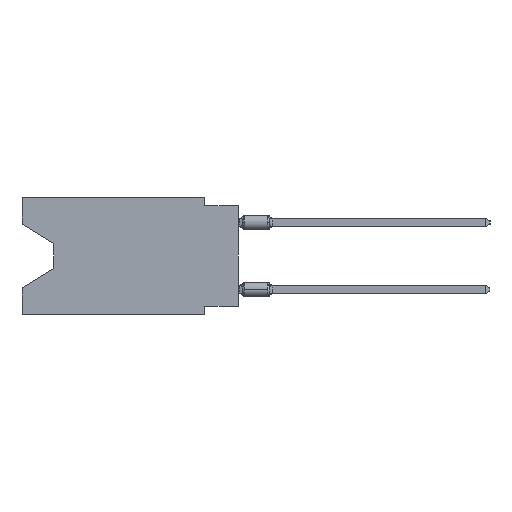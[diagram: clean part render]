
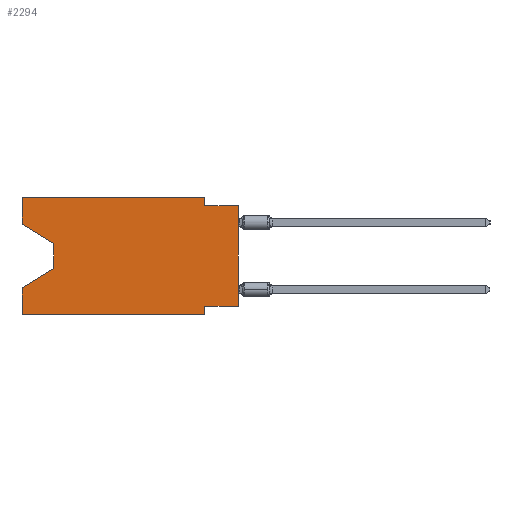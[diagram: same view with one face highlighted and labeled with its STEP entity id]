
A CAD part, left-side view. The second image highlights one B-rep face of the part: STEP entity #2294.
In plain terms, the highlighted planar face has unit normal (-1, 0, 0).
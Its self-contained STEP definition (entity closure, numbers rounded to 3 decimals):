
#181 = ORIENTED_EDGE ( 'NONE', *, *, #17903, .F. ) ;
#265 = LINE ( 'NONE', #28684, #13404 ) ;
#426 = VERTEX_POINT ( 'NONE', #13703 ) ;
#1508 = EDGE_CURVE ( 'NONE', #11609, #426, #4646, .T. ) ;
#1992 = ORIENTED_EDGE ( 'NONE', *, *, #17382, .T. ) ;
#2086 = ORIENTED_EDGE ( 'NONE', *, *, #25789, .F. ) ;
#2294 = ADVANCED_FACE ( 'NONE', ( #4104 ), #13522, .F. ) ;
#2519 = CARTESIAN_POINT ( 'NONE',  ( 0., 16.383, -8.89 ) ) ;
#3212 = VERTEX_POINT ( 'NONE', #23504 ) ;
#3384 = EDGE_CURVE ( 'NONE', #19287, #3212, #8581, .T. ) ;
#4104 = FACE_OUTER_BOUND ( 'NONE', #4365, .T. ) ;
#4188 = EDGE_CURVE ( 'NONE', #10632, #11609, #29544, .T. ) ;
#4365 = EDGE_LOOP ( 'NONE', ( #20825, #10486, #22707, #2086, #10446, #16265, #16958, #1992, #13049, #181, #12769, #13996 ) ) ;
#4429 = CARTESIAN_POINT ( 'NONE',  ( 0., 0., -8.255 ) ) ;
#4646 = LINE ( 'NONE', #26424, #22206 ) ;
#5710 = VERTEX_POINT ( 'NONE', #7734 ) ;
#6050 = CARTESIAN_POINT ( 'NONE',  ( 0., 13.97, -3.505 ) ) ;
#6409 = CARTESIAN_POINT ( 'NONE',  ( 0., 16.383, 0. ) ) ;
#6867 = VERTEX_POINT ( 'NONE', #6409 ) ;
#7337 = DIRECTION ( 'NONE',  ( 0., 0., -1. ) ) ;
#7412 = DIRECTION ( 'NONE',  ( 0., 0.855, -0.519 ) ) ;
#7734 = CARTESIAN_POINT ( 'NONE',  ( 0., 2.54, -0.635 ) ) ;
#8309 = VECTOR ( 'NONE', #18363, 1000. ) ;
#8549 = LINE ( 'NONE', #27427, #27385 ) ;
#8566 = EDGE_CURVE ( 'NONE', #23685, #6867, #21553, .T. ) ;
#8581 = LINE ( 'NONE', #22816, #19250 ) ;
#10019 = CARTESIAN_POINT ( 'NONE',  ( 0., 0., -0.635 ) ) ;
#10324 = LINE ( 'NONE', #10019, #10648 ) ;
#10446 = ORIENTED_EDGE ( 'NONE', *, *, #27778, .T. ) ;
#10486 = ORIENTED_EDGE ( 'NONE', *, *, #4188, .T. ) ;
#10632 = VERTEX_POINT ( 'NONE', #27458 ) ;
#10648 = VECTOR ( 'NONE', #22377, 1000. ) ;
#10943 = LINE ( 'NONE', #29951, #8309 ) ;
#11191 = CARTESIAN_POINT ( 'NONE',  ( 0., 2.54, 0. ) ) ;
#11609 = VERTEX_POINT ( 'NONE', #29880 ) ;
#11934 = DIRECTION ( 'NONE',  ( 0., -1., 0. ) ) ;
#12244 = LINE ( 'NONE', #22530, #25513 ) ;
#12429 = CARTESIAN_POINT ( 'NONE',  ( 0., 16.383, 0. ) ) ;
#12695 = VERTEX_POINT ( 'NONE', #29581 ) ;
#12769 = ORIENTED_EDGE ( 'NONE', *, *, #14696, .F. ) ;
#12809 = VECTOR ( 'NONE', #20206, 1000. ) ;
#13049 = ORIENTED_EDGE ( 'NONE', *, *, #26708, .F. ) ;
#13112 = CARTESIAN_POINT ( 'NONE',  ( 0., 2.54, -8.255 ) ) ;
#13404 = VECTOR ( 'NONE', #21269, 1000. ) ;
#13522 = PLANE ( 'NONE',  #30072 ) ;
#13703 = CARTESIAN_POINT ( 'NONE',  ( 0., 16.383, -6.852 ) ) ;
#13996 = ORIENTED_EDGE ( 'NONE', *, *, #8566, .F. ) ;
#14696 = EDGE_CURVE ( 'NONE', #6867, #26995, #10943, .T. ) ;
#16265 = ORIENTED_EDGE ( 'NONE', *, *, #3384, .F. ) ;
#16958 = ORIENTED_EDGE ( 'NONE', *, *, #27946, .F. ) ;
#17382 = EDGE_CURVE ( 'NONE', #22480, #12695, #17740, .T. ) ;
#17740 = LINE ( 'NONE', #27169, #12809 ) ;
#17895 = DIRECTION ( 'NONE',  ( 0., 1., 0. ) ) ;
#17903 = EDGE_CURVE ( 'NONE', #26995, #5710, #23094, .T. ) ;
#17956 = DIRECTION ( 'NONE',  ( 0., 0., -1. ) ) ;
#18363 = DIRECTION ( 'NONE',  ( 0., -1., 0. ) ) ;
#18827 = CARTESIAN_POINT ( 'NONE',  ( 0., 16.383, -2.038 ) ) ;
#19250 = VECTOR ( 'NONE', #27456, 1000. ) ;
#19287 = VERTEX_POINT ( 'NONE', #13112 ) ;
#19918 = EDGE_CURVE ( 'NONE', #23685, #10632, #265, .T. ) ;
#20206 = DIRECTION ( 'NONE',  ( 0., 0., 1. ) ) ;
#20247 = VERTEX_POINT ( 'NONE', #25097 ) ;
#20254 = VECTOR ( 'NONE', #17956, 1000. ) ;
#20321 = DIRECTION ( 'NONE',  ( 0., 0., -1. ) ) ;
#20825 = ORIENTED_EDGE ( 'NONE', *, *, #19918, .T. ) ;
#21269 = DIRECTION ( 'NONE',  ( 0., -0.855, -0.519 ) ) ;
#21474 = VECTOR ( 'NONE', #21854, 1000. ) ;
#21553 = LINE ( 'NONE', #12429, #21474 ) ;
#21854 = DIRECTION ( 'NONE',  ( 0., 0., 1. ) ) ;
#22206 = VECTOR ( 'NONE', #7412, 1000. ) ;
#22377 = DIRECTION ( 'NONE',  ( 0., -1., 0. ) ) ;
#22480 = VERTEX_POINT ( 'NONE', #4429 ) ;
#22530 = CARTESIAN_POINT ( 'NONE',  ( 0., 0., -8.255 ) ) ;
#22545 = VECTOR ( 'NONE', #11934, 1000. ) ;
#22707 = ORIENTED_EDGE ( 'NONE', *, *, #1508, .T. ) ;
#22708 = VECTOR ( 'NONE', #20321, 1000. ) ;
#22816 = CARTESIAN_POINT ( 'NONE',  ( 0., 2.54, -8.89 ) ) ;
#23094 = LINE ( 'NONE', #11191, #22708 ) ;
#23410 = CARTESIAN_POINT ( 'NONE',  ( 0., 16.383, 0. ) ) ;
#23504 = CARTESIAN_POINT ( 'NONE',  ( 0., 2.54, -8.89 ) ) ;
#23685 = VERTEX_POINT ( 'NONE', #18827 ) ;
#23908 = CARTESIAN_POINT ( 'NONE',  ( 0., 2.54, 0. ) ) ;
#24797 = DIRECTION ( 'NONE',  ( 0., 0., 1. ) ) ;
#25097 = CARTESIAN_POINT ( 'NONE',  ( 0., 16.383, -8.89 ) ) ;
#25513 = VECTOR ( 'NONE', #17895, 1000. ) ;
#25789 = EDGE_CURVE ( 'NONE', #20247, #426, #8549, .T. ) ;
#25848 = LINE ( 'NONE', #2519, #22545 ) ;
#26424 = CARTESIAN_POINT ( 'NONE',  ( 0., 13.97, -5.385 ) ) ;
#26708 = EDGE_CURVE ( 'NONE', #5710, #12695, #10324, .T. ) ;
#26995 = VERTEX_POINT ( 'NONE', #23908 ) ;
#27169 = CARTESIAN_POINT ( 'NONE',  ( 0., 0., 0. ) ) ;
#27385 = VECTOR ( 'NONE', #24797, 1000. ) ;
#27427 = CARTESIAN_POINT ( 'NONE',  ( 0., 16.383, 0. ) ) ;
#27456 = DIRECTION ( 'NONE',  ( 0., 0., -1. ) ) ;
#27458 = CARTESIAN_POINT ( 'NONE',  ( 0., 13.97, -3.505 ) ) ;
#27778 = EDGE_CURVE ( 'NONE', #20247, #3212, #25848, .T. ) ;
#27946 = EDGE_CURVE ( 'NONE', #22480, #19287, #12244, .T. ) ;
#28520 = DIRECTION ( 'NONE',  ( 1., 0., 0. ) ) ;
#28684 = CARTESIAN_POINT ( 'NONE',  ( 0., 16.383, -2.038 ) ) ;
#29544 = LINE ( 'NONE', #6050, #20254 ) ;
#29581 = CARTESIAN_POINT ( 'NONE',  ( 0., 0., -0.635 ) ) ;
#29880 = CARTESIAN_POINT ( 'NONE',  ( 0., 13.97, -5.385 ) ) ;
#29951 = CARTESIAN_POINT ( 'NONE',  ( 0., 16.383, 0. ) ) ;
#30072 = AXIS2_PLACEMENT_3D ( 'NONE', #23410, #28520, #7337 ) ;
